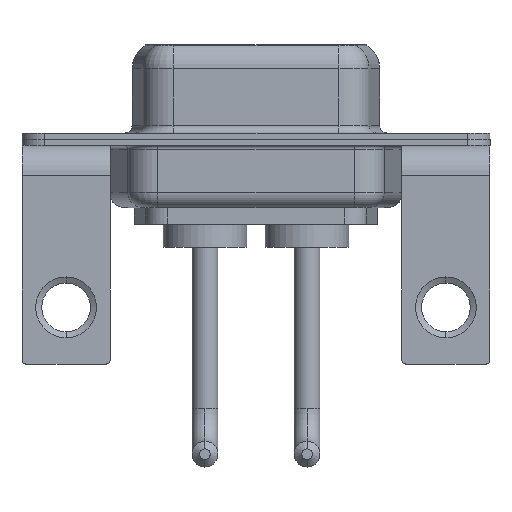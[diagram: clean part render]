
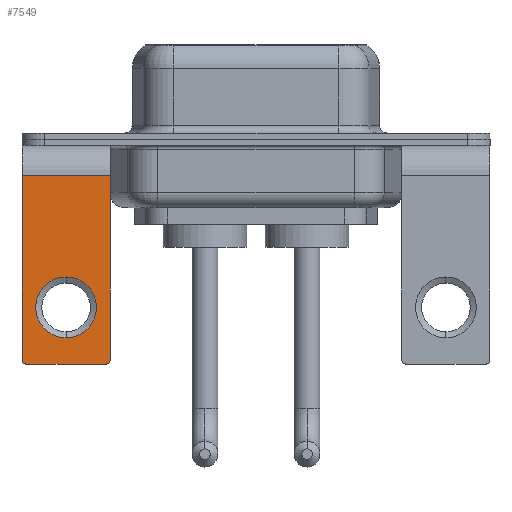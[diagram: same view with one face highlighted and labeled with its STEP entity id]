
A CAD part, front view. The second image highlights one B-rep face of the part: STEP entity #7549.
In plain terms, the highlighted planar face has unit normal (0, -1, 0).
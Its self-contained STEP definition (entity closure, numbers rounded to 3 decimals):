
#424 = DIRECTION ( 'NONE',  ( -1., 0., 0. ) ) ;
#441 = DIRECTION ( 'NONE',  ( 0., 0., -1. ) ) ;
#569 = CARTESIAN_POINT ( 'NONE',  ( 2.9, -6.25, -2.4 ) ) ;
#681 = CARTESIAN_POINT ( 'NONE',  ( 2.9, -6.25, -2.4 ) ) ;
#1519 = VERTEX_POINT ( 'NONE', #11091 ) ;
#1983 = ORIENTED_EDGE ( 'NONE', *, *, #7620, .T. ) ;
#2078 = EDGE_CURVE ( 'NONE', #3426, #1519, #11076, .T. ) ;
#2087 = CIRCLE ( 'NONE', #7087, 0.25 ) ;
#2119 = AXIS2_PLACEMENT_3D ( 'NONE', #10400, #9557, #5626 ) ;
#2436 = VERTEX_POINT ( 'NONE', #7304 ) ;
#2833 = DIRECTION ( 'NONE',  ( 0., 1., 0. ) ) ;
#2962 = CARTESIAN_POINT ( 'NONE',  ( 0., -6.25, -11.07 ) ) ;
#3134 = CIRCLE ( 'NONE', #9411, 2. ) ;
#3145 = VECTOR ( 'NONE', #8153, 1000. ) ;
#3154 = CARTESIAN_POINT ( 'NONE',  ( 2.65, -6.25, -14.55 ) ) ;
#3158 = VERTEX_POINT ( 'NONE', #681 ) ;
#3220 = CARTESIAN_POINT ( 'NONE',  ( 2.65, -6.25, -14.8 ) ) ;
#3426 = VERTEX_POINT ( 'NONE', #3220 ) ;
#3512 = LINE ( 'NONE', #569, #12082 ) ;
#3539 = AXIS2_PLACEMENT_3D ( 'NONE', #7107, #4988, #4919 ) ;
#3794 = CARTESIAN_POINT ( 'NONE',  ( -2.9, -6.25, -14.55 ) ) ;
#4083 = DIRECTION ( 'NONE',  ( 0., 1., 0. ) ) ;
#4176 = CARTESIAN_POINT ( 'NONE',  ( -2.9, -6.25, -2.4 ) ) ;
#4362 = CIRCLE ( 'NONE', #3539, 2. ) ;
#4513 = VECTOR ( 'NONE', #424, 1000. ) ;
#4558 = EDGE_CURVE ( 'NONE', #3158, #12035, #4655, .T. ) ;
#4655 = LINE ( 'NONE', #7712, #6644 ) ;
#4680 = EDGE_LOOP ( 'NONE', ( #1983, #6977 ) ) ;
#4742 = EDGE_CURVE ( 'NONE', #5448, #10468, #4362, .T. ) ;
#4801 = DIRECTION ( 'NONE',  ( 0., 0., 1. ) ) ;
#4919 = DIRECTION ( 'NONE',  ( 0., 0., 1. ) ) ;
#4988 = DIRECTION ( 'NONE',  ( 0., 1., 0. ) ) ;
#5006 = CARTESIAN_POINT ( 'NONE',  ( 2.9, -6.25, -2.4 ) ) ;
#5032 = VERTEX_POINT ( 'NONE', #3794 ) ;
#5269 = ORIENTED_EDGE ( 'NONE', *, *, #7727, .T. ) ;
#5448 = VERTEX_POINT ( 'NONE', #5737 ) ;
#5547 = CARTESIAN_POINT ( 'NONE',  ( 0., -6.25, -13.07 ) ) ;
#5626 = DIRECTION ( 'NONE',  ( 0., 0., 1. ) ) ;
#5638 = DIRECTION ( 'NONE',  ( -1., 0., 0. ) ) ;
#5737 = CARTESIAN_POINT ( 'NONE',  ( 0., -6.25, -9.07 ) ) ;
#5942 = LINE ( 'NONE', #4176, #3145 ) ;
#5973 = PLANE ( 'NONE',  #8985 ) ;
#6098 = EDGE_LOOP ( 'NONE', ( #8535, #11206, #11602, #5269, #11467, #10483 ) ) ;
#6106 = CARTESIAN_POINT ( 'NONE',  ( 2.9, -6.25, -14.8 ) ) ;
#6287 = DIRECTION ( 'NONE',  ( 0., -1., 0. ) ) ;
#6531 = EDGE_CURVE ( 'NONE', #12035, #5032, #5942, .T. ) ;
#6644 = VECTOR ( 'NONE', #5638, 1000. ) ;
#6872 = DIRECTION ( 'NONE',  ( 0., 0., 1. ) ) ;
#6977 = ORIENTED_EDGE ( 'NONE', *, *, #4742, .T. ) ;
#6999 = FACE_OUTER_BOUND ( 'NONE', #6098, .T. ) ;
#7087 = AXIS2_PLACEMENT_3D ( 'NONE', #3154, #6287, #11317 ) ;
#7107 = CARTESIAN_POINT ( 'NONE',  ( 0., -6.25, -11.07 ) ) ;
#7304 = CARTESIAN_POINT ( 'NONE',  ( 2.9, -6.25, -14.55 ) ) ;
#7549 = ADVANCED_FACE ( 'NONE', ( #12917, #6999 ), #5973, .F. ) ;
#7620 = EDGE_CURVE ( 'NONE', #10468, #5448, #3134, .T. ) ;
#7712 = CARTESIAN_POINT ( 'NONE',  ( 2.9, -6.25, -2.4 ) ) ;
#7727 = EDGE_CURVE ( 'NONE', #3426, #2436, #2087, .T. ) ;
#7750 = CIRCLE ( 'NONE', #2119, 0.25 ) ;
#8153 = DIRECTION ( 'NONE',  ( 0., 0., -1. ) ) ;
#8266 = EDGE_CURVE ( 'NONE', #5032, #1519, #7750, .T. ) ;
#8535 = ORIENTED_EDGE ( 'NONE', *, *, #6531, .T. ) ;
#8643 = CARTESIAN_POINT ( 'NONE',  ( -2.9, -6.25, -2.4 ) ) ;
#8985 = AXIS2_PLACEMENT_3D ( 'NONE', #5006, #2833, #4801 ) ;
#9411 = AXIS2_PLACEMENT_3D ( 'NONE', #2962, #4083, #6872 ) ;
#9557 = DIRECTION ( 'NONE',  ( 0., -1., 0. ) ) ;
#10400 = CARTESIAN_POINT ( 'NONE',  ( -2.65, -6.25, -14.55 ) ) ;
#10468 = VERTEX_POINT ( 'NONE', #5547 ) ;
#10483 = ORIENTED_EDGE ( 'NONE', *, *, #4558, .T. ) ;
#10937 = EDGE_CURVE ( 'NONE', #3158, #2436, #3512, .T. ) ;
#11076 = LINE ( 'NONE', #6106, #4513 ) ;
#11091 = CARTESIAN_POINT ( 'NONE',  ( -2.65, -6.25, -14.8 ) ) ;
#11206 = ORIENTED_EDGE ( 'NONE', *, *, #8266, .T. ) ;
#11317 = DIRECTION ( 'NONE',  ( 0., 0., 1. ) ) ;
#11467 = ORIENTED_EDGE ( 'NONE', *, *, #10937, .F. ) ;
#11602 = ORIENTED_EDGE ( 'NONE', *, *, #2078, .F. ) ;
#12035 = VERTEX_POINT ( 'NONE', #8643 ) ;
#12082 = VECTOR ( 'NONE', #441, 1000. ) ;
#12917 = FACE_BOUND ( 'NONE', #4680, .T. ) ;
